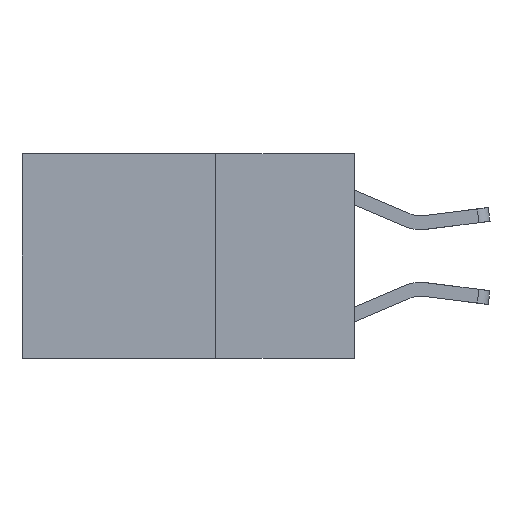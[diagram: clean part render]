
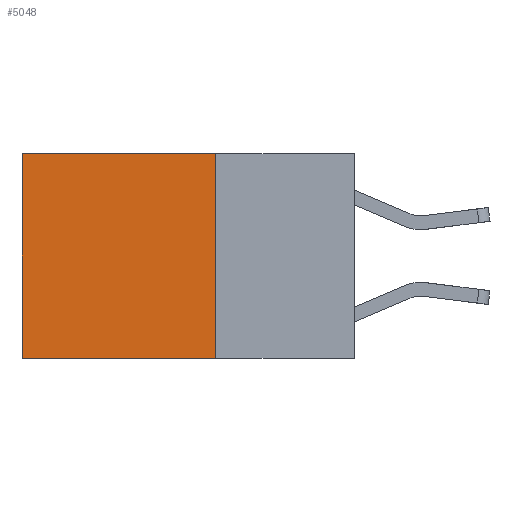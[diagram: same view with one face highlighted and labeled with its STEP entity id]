
A CAD part, left-side view. The second image highlights one B-rep face of the part: STEP entity #5048.
In plain terms, the highlighted planar face has unit normal (-1, 0, 0).
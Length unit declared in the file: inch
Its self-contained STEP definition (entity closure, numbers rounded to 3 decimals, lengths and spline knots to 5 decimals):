
#175 = CARTESIAN_POINT ( 'NONE',  ( 0.2625, 0.6, 0. ) ) ;
#379 = VERTEX_POINT ( 'NONE', #8766 ) ;
#627 = DIRECTION ( 'NONE',  ( 0., 1., 0. ) ) ;
#1015 = CARTESIAN_POINT ( 'NONE',  ( 0.2625, 0.25, 0. ) ) ;
#1713 = VERTEX_POINT ( 'NONE', #10907 ) ;
#1828 = DIRECTION ( 'NONE',  ( 0., 0., -1. ) ) ;
#2376 = VECTOR ( 'NONE', #1828, 39.37008 ) ;
#2825 = VECTOR ( 'NONE', #10245, 39.37008 ) ;
#3081 = LINE ( 'NONE', #7532, #6437 ) ;
#3310 = DIRECTION ( 'NONE',  ( 1., 0., 0. ) ) ;
#3340 = EDGE_CURVE ( 'NONE', #8439, #5651, #4083, .T. ) ;
#4083 = LINE ( 'NONE', #6730, #2825 ) ;
#4979 = ORIENTED_EDGE ( 'NONE', *, *, #11122, .F. ) ;
#5048 = ADVANCED_FACE ( 'NONE', ( #7644 ), #7472, .F. ) ;
#5651 = VERTEX_POINT ( 'NONE', #8691 ) ;
#5884 = CARTESIAN_POINT ( 'NONE',  ( 0.2625, 0.25, 0. ) ) ;
#6395 = AXIS2_PLACEMENT_3D ( 'NONE', #5884, #3310, #7590 ) ;
#6437 = VECTOR ( 'NONE', #627, 39.37008 ) ;
#6730 = CARTESIAN_POINT ( 'NONE',  ( 0.2625, 0.25, -0.37 ) ) ;
#7230 = LINE ( 'NONE', #1015, #9207 ) ;
#7472 = PLANE ( 'NONE',  #6395 ) ;
#7532 = CARTESIAN_POINT ( 'NONE',  ( 0.2625, 0.25, 0. ) ) ;
#7590 = DIRECTION ( 'NONE',  ( 0., 0., -1. ) ) ;
#7644 = FACE_OUTER_BOUND ( 'NONE', #8096, .T. ) ;
#7885 = ORIENTED_EDGE ( 'NONE', *, *, #10831, .T. ) ;
#8096 = EDGE_LOOP ( 'NONE', ( #10867, #10727, #4979, #7885 ) ) ;
#8439 = VERTEX_POINT ( 'NONE', #9195 ) ;
#8691 = CARTESIAN_POINT ( 'NONE',  ( 0.2625, 0.6, -0.37 ) ) ;
#8766 = CARTESIAN_POINT ( 'NONE',  ( 0.2625, 0.6, 0. ) ) ;
#8820 = LINE ( 'NONE', #175, #2376 ) ;
#9195 = CARTESIAN_POINT ( 'NONE',  ( 0.2625, 0.25, -0.37 ) ) ;
#9207 = VECTOR ( 'NONE', #10773, 39.37008 ) ;
#9465 = EDGE_CURVE ( 'NONE', #379, #5651, #8820, .T. ) ;
#10245 = DIRECTION ( 'NONE',  ( 0., 1., 0. ) ) ;
#10727 = ORIENTED_EDGE ( 'NONE', *, *, #3340, .F. ) ;
#10773 = DIRECTION ( 'NONE',  ( 0., 0., -1. ) ) ;
#10831 = EDGE_CURVE ( 'NONE', #1713, #379, #3081, .T. ) ;
#10867 = ORIENTED_EDGE ( 'NONE', *, *, #9465, .T. ) ;
#10907 = CARTESIAN_POINT ( 'NONE',  ( 0.2625, 0.25, 0. ) ) ;
#11122 = EDGE_CURVE ( 'NONE', #1713, #8439, #7230, .T. ) ;
